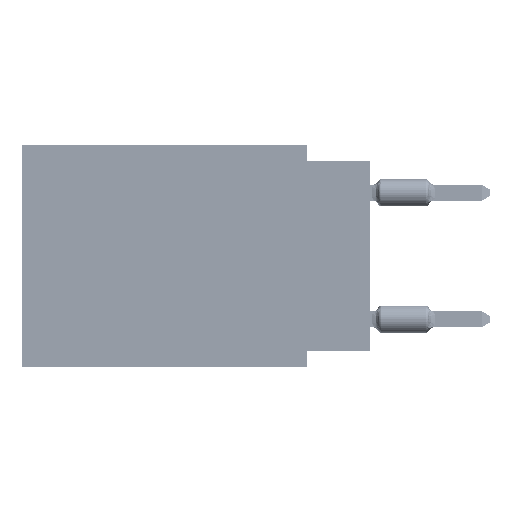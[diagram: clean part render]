
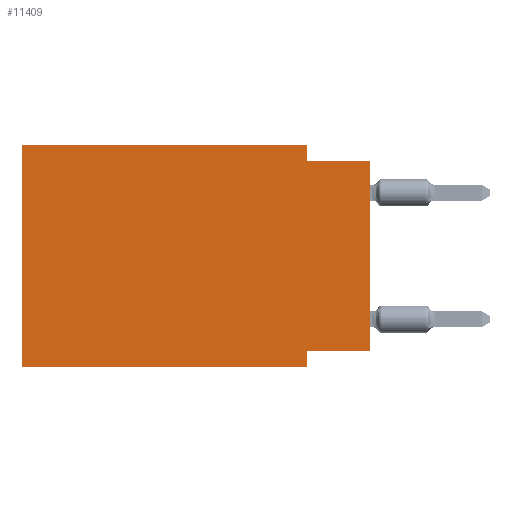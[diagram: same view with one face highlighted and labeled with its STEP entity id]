
A CAD part, left-side view. The second image highlights one B-rep face of the part: STEP entity #11409.
In plain terms, the highlighted planar face has unit normal (-1, 0, 0).
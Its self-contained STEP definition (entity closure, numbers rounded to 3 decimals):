
#456 = DIRECTION ( 'NONE',  ( 0., 0., -1. ) ) ;
#1134 = CARTESIAN_POINT ( 'NONE',  ( 0., 13.97, 0. ) ) ;
#1940 = CARTESIAN_POINT ( 'NONE',  ( 0., 2.54, -0.635 ) ) ;
#2952 = EDGE_CURVE ( 'NONE', #20162, #29999, #60376, .T. ) ;
#3915 = DIRECTION ( 'NONE',  ( 0., -1., 0. ) ) ;
#5642 = DIRECTION ( 'NONE',  ( 0., 0., 1. ) ) ;
#6439 = LINE ( 'NONE', #36162, #54751 ) ;
#6475 = VECTOR ( 'NONE', #33922, 1000. ) ;
#9103 = ORIENTED_EDGE ( 'NONE', *, *, #2952, .F. ) ;
#11161 = LINE ( 'NONE', #1134, #15054 ) ;
#11409 = ADVANCED_FACE ( 'NONE', ( #37452 ), #52497, .F. ) ;
#12429 = VERTEX_POINT ( 'NONE', #19483 ) ;
#12713 = DIRECTION ( 'NONE',  ( 0., 0., -1. ) ) ;
#13551 = CARTESIAN_POINT ( 'NONE',  ( 0., 2.54, 0. ) ) ;
#14397 = VECTOR ( 'NONE', #5642, 1000. ) ;
#15054 = VECTOR ( 'NONE', #30851, 1000. ) ;
#15192 = EDGE_CURVE ( 'NONE', #37519, #63134, #11161, .T. ) ;
#16004 = LINE ( 'NONE', #48378, #46094 ) ;
#16350 = LINE ( 'NONE', #31014, #14397 ) ;
#19457 = CARTESIAN_POINT ( 'NONE',  ( 0., 0., -8.255 ) ) ;
#19483 = CARTESIAN_POINT ( 'NONE',  ( 0., 2.54, -8.89 ) ) ;
#20105 = VERTEX_POINT ( 'NONE', #23284 ) ;
#20162 = VERTEX_POINT ( 'NONE', #1940 ) ;
#20327 = CARTESIAN_POINT ( 'NONE',  ( 0., 13.97, 0. ) ) ;
#21028 = ORIENTED_EDGE ( 'NONE', *, *, #42399, .F. ) ;
#21545 = ORIENTED_EDGE ( 'NONE', *, *, #38954, .F. ) ;
#22739 = CARTESIAN_POINT ( 'NONE',  ( 0., 0., -0.635 ) ) ;
#22764 = DIRECTION ( 'NONE',  ( 0., -1., 0. ) ) ;
#23284 = CARTESIAN_POINT ( 'NONE',  ( 0., 2.54, 0. ) ) ;
#24803 = LINE ( 'NONE', #19457, #58362 ) ;
#26420 = ORIENTED_EDGE ( 'NONE', *, *, #15192, .F. ) ;
#29999 = VERTEX_POINT ( 'NONE', #22739 ) ;
#30851 = DIRECTION ( 'NONE',  ( 0., 0., 1. ) ) ;
#31014 = CARTESIAN_POINT ( 'NONE',  ( 0., 0., 0. ) ) ;
#32999 = EDGE_CURVE ( 'NONE', #37519, #12429, #48109, .T. ) ;
#33014 = DIRECTION ( 'NONE',  ( 0., -1., 0. ) ) ;
#33356 = VERTEX_POINT ( 'NONE', #46388 ) ;
#33436 = CARTESIAN_POINT ( 'NONE',  ( 0., 13.97, -8.89 ) ) ;
#33445 = CARTESIAN_POINT ( 'NONE',  ( 0., 13.97, 0. ) ) ;
#33922 = DIRECTION ( 'NONE',  ( 0., 0., -1. ) ) ;
#34870 = VECTOR ( 'NONE', #22764, 1000. ) ;
#36162 = CARTESIAN_POINT ( 'NONE',  ( 0., 2.54, -8.89 ) ) ;
#37452 = FACE_OUTER_BOUND ( 'NONE', #43668, .T. ) ;
#37519 = VERTEX_POINT ( 'NONE', #64252 ) ;
#38954 = EDGE_CURVE ( 'NONE', #63134, #20105, #16004, .T. ) ;
#42399 = EDGE_CURVE ( 'NONE', #20105, #20162, #59324, .T. ) ;
#43668 = EDGE_LOOP ( 'NONE', ( #45975, #9103, #21028, #21545, #26420, #64897, #52611, #51798 ) ) ;
#45676 = VERTEX_POINT ( 'NONE', #62655 ) ;
#45975 = ORIENTED_EDGE ( 'NONE', *, *, #56832, .T. ) ;
#46094 = VECTOR ( 'NONE', #33014, 1000. ) ;
#46388 = CARTESIAN_POINT ( 'NONE',  ( 0., 2.54, -8.255 ) ) ;
#48109 = LINE ( 'NONE', #33436, #34870 ) ;
#48378 = CARTESIAN_POINT ( 'NONE',  ( 0., 13.97, 0. ) ) ;
#48941 = VECTOR ( 'NONE', #3915, 1000. ) ;
#50357 = CARTESIAN_POINT ( 'NONE',  ( 0., 0., -0.635 ) ) ;
#51798 = ORIENTED_EDGE ( 'NONE', *, *, #59371, .F. ) ;
#52497 = PLANE ( 'NONE',  #61951 ) ;
#52611 = ORIENTED_EDGE ( 'NONE', *, *, #54729, .F. ) ;
#54729 = EDGE_CURVE ( 'NONE', #33356, #12429, #6439, .T. ) ;
#54751 = VECTOR ( 'NONE', #456, 1000. ) ;
#54851 = DIRECTION ( 'NONE',  ( 0., 1., 0. ) ) ;
#56832 = EDGE_CURVE ( 'NONE', #45676, #29999, #16350, .T. ) ;
#58173 = DIRECTION ( 'NONE',  ( 1., 0., 0. ) ) ;
#58362 = VECTOR ( 'NONE', #54851, 1000. ) ;
#59324 = LINE ( 'NONE', #13551, #6475 ) ;
#59371 = EDGE_CURVE ( 'NONE', #45676, #33356, #24803, .T. ) ;
#60376 = LINE ( 'NONE', #50357, #48941 ) ;
#61951 = AXIS2_PLACEMENT_3D ( 'NONE', #33445, #58173, #12713 ) ;
#62655 = CARTESIAN_POINT ( 'NONE',  ( 0., 0., -8.255 ) ) ;
#63134 = VERTEX_POINT ( 'NONE', #20327 ) ;
#64252 = CARTESIAN_POINT ( 'NONE',  ( 0., 13.97, -8.89 ) ) ;
#64897 = ORIENTED_EDGE ( 'NONE', *, *, #32999, .T. ) ;
